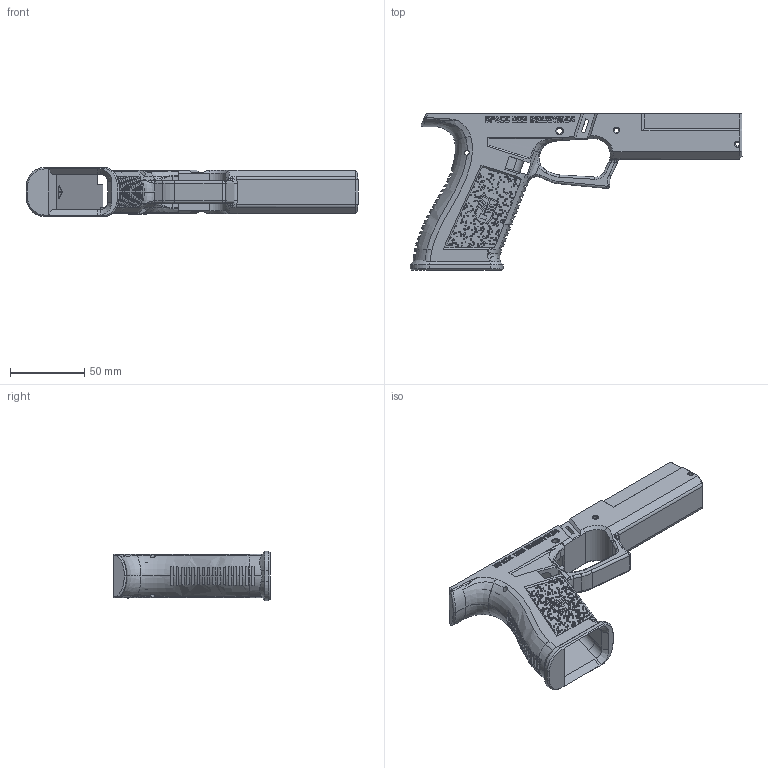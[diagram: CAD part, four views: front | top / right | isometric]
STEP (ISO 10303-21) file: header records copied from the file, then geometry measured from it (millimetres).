
FILE_DESCRIPTION(/* description */ (''),/* implementation_level */ '2;1');
FILE_NAME(/* name */ 'PY2A SDI GXL34 Competition FM.step',/* time_stamp */ '2022-06-26T09:14:13-05:00',/* author */ (''),/* organization */ (''),/* preprocessor_version */ 'ST-DEVELOPER v19',/* originating_system */ 'Autodesk Translation Framework v11.7.0.108',/* authorisation */ '');
FILE_SCHEMA (('AUTOMOTIVE_DESIGN { 1 0 10303 214 3 1 1 }'));
Products named in the file (1): PY2A SDI GXL Competition
Bounding box: 223.95 x 105.56 x 33.23 mm (x, y, z)
Volume: 136800.9 mm3; surface area: 60861.2 mm2
Topology: 1 solids, 2 shells, 3422 faces, 8883 edges, 5859 vertices
Faces by surface type: bspline 2349, plane 1004, cylinder 56, torus 7, cone 6
Full cylindrical faces by diameter (mm): 1.933 x1, 3 x2, 3.05 x2, 3.146 x2, 3.5 x1, 4.1 x2, 14 x1
Entity records: 138452 total; most frequent: CARTESIAN_POINT 77703, ORIENTED_EDGE 17754, EDGE_CURVE 8877, DIRECTION 6087, VERTEX_POINT 5859, EDGE_LOOP 3854, LINE 3567, VECTOR 3567
